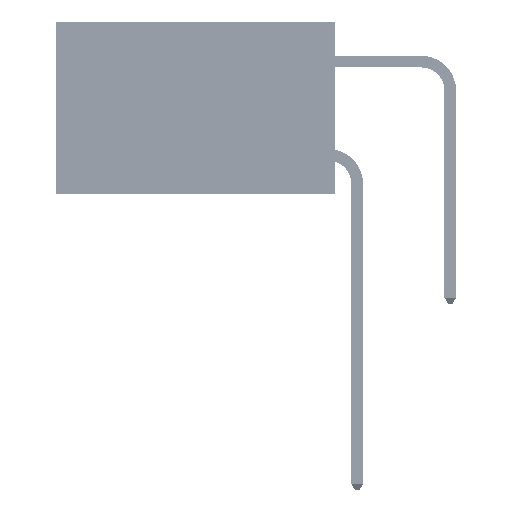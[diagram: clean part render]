
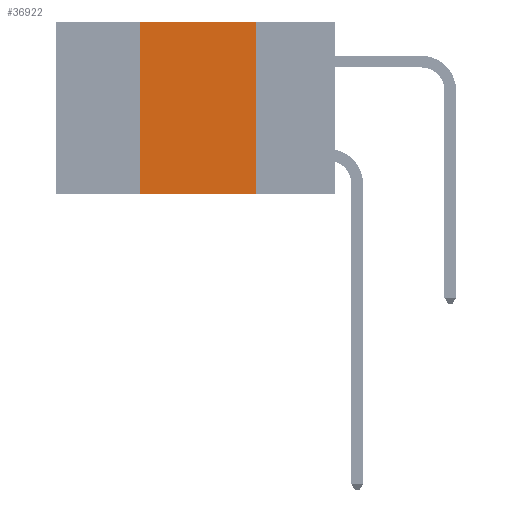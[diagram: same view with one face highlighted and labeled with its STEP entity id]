
A CAD part, left-side view. The second image highlights one B-rep face of the part: STEP entity #36922.
In plain terms, the highlighted planar face has unit normal (-1, 0, 0).
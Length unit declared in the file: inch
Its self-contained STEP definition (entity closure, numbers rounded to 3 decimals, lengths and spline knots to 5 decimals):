
#764 = DIRECTION ( 'NONE',  ( 0., 0., -1. ) ) ;
#907 = VERTEX_POINT ( 'NONE', #37773 ) ;
#3239 = EDGE_CURVE ( 'NONE', #24133, #30958, #39471, .T. ) ;
#6099 = CARTESIAN_POINT ( 'NONE',  ( 0., 0.42, 0. ) ) ;
#6278 = EDGE_CURVE ( 'NONE', #907, #19420, #28769, .T. ) ;
#6519 = CARTESIAN_POINT ( 'NONE',  ( 0., 0.17, 0. ) ) ;
#7893 = CARTESIAN_POINT ( 'NONE',  ( 0., 0.17, -0.37 ) ) ;
#8441 = CARTESIAN_POINT ( 'NONE',  ( 0., 0.6, 0. ) ) ;
#9523 = CARTESIAN_POINT ( 'NONE',  ( 0., 0.42, 0. ) ) ;
#10231 = EDGE_CURVE ( 'NONE', #30958, #907, #37010, .T. ) ;
#11011 = DIRECTION ( 'NONE',  ( 0., -1., 0. ) ) ;
#12445 = LINE ( 'NONE', #22084, #46852 ) ;
#12915 = DIRECTION ( 'NONE',  ( 0., 0., 1. ) ) ;
#13188 = AXIS2_PLACEMENT_3D ( 'NONE', #8441, #45932, #764 ) ;
#16496 = ORIENTED_EDGE ( 'NONE', *, *, #6278, .F. ) ;
#16639 = FACE_OUTER_BOUND ( 'NONE', #28272, .T. ) ;
#19420 = VERTEX_POINT ( 'NONE', #7893 ) ;
#20331 = ORIENTED_EDGE ( 'NONE', *, *, #10231, .F. ) ;
#21649 = DIRECTION ( 'NONE',  ( 0., 0., -1. ) ) ;
#22084 = CARTESIAN_POINT ( 'NONE',  ( 0., 0.6, -0.37 ) ) ;
#22630 = CARTESIAN_POINT ( 'NONE',  ( 0., 0.6, 0. ) ) ;
#24133 = VERTEX_POINT ( 'NONE', #47306 ) ;
#25929 = VECTOR ( 'NONE', #25934, 39.37008 ) ;
#25934 = DIRECTION ( 'NONE',  ( 0., -1., 0. ) ) ;
#28272 = EDGE_LOOP ( 'NONE', ( #16496, #20331, #42413, #30844 ) ) ;
#28769 = LINE ( 'NONE', #6519, #47385 ) ;
#30844 = ORIENTED_EDGE ( 'NONE', *, *, #31776, .T. ) ;
#30958 = VERTEX_POINT ( 'NONE', #9523 ) ;
#31776 = EDGE_CURVE ( 'NONE', #24133, #19420, #12445, .T. ) ;
#31923 = VECTOR ( 'NONE', #12915, 39.37008 ) ;
#34245 = PLANE ( 'NONE',  #13188 ) ;
#36922 = ADVANCED_FACE ( 'NONE', ( #16639 ), #34245, .F. ) ;
#37010 = LINE ( 'NONE', #22630, #25929 ) ;
#37773 = CARTESIAN_POINT ( 'NONE',  ( 0., 0.17, 0. ) ) ;
#39471 = LINE ( 'NONE', #6099, #31923 ) ;
#42413 = ORIENTED_EDGE ( 'NONE', *, *, #3239, .F. ) ;
#45932 = DIRECTION ( 'NONE',  ( 1., 0., 0. ) ) ;
#46852 = VECTOR ( 'NONE', #11011, 39.37008 ) ;
#47306 = CARTESIAN_POINT ( 'NONE',  ( 0., 0.42, -0.37 ) ) ;
#47385 = VECTOR ( 'NONE', #21649, 39.37008 ) ;
